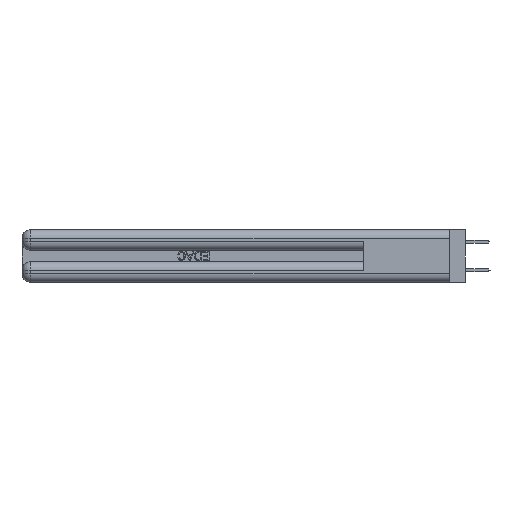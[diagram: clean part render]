
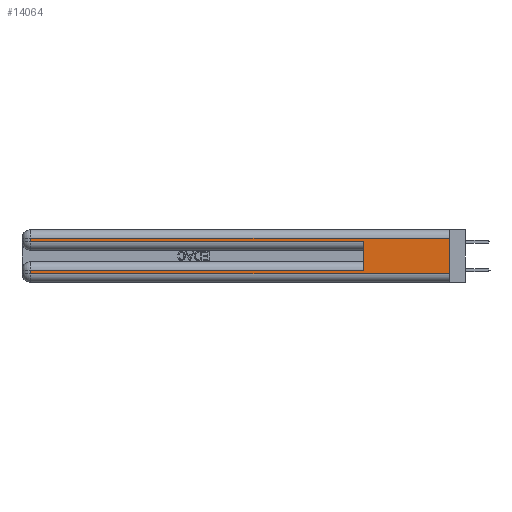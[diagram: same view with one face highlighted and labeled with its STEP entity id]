
A CAD part, left-side view. The second image highlights one B-rep face of the part: STEP entity #14064.
In plain terms, the highlighted planar face has unit normal (-1, 0, 0).
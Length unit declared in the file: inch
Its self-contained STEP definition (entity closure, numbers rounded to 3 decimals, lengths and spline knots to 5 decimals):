
#361 = DIRECTION ( 'NONE',  ( 0., 0., -1. ) ) ;
#1210 = LINE ( 'NONE', #43359, #11063 ) ;
#1530 = CARTESIAN_POINT ( 'NONE',  ( 0., 2.94, 0.31 ) ) ;
#2411 = VERTEX_POINT ( 'NONE', #1530 ) ;
#2597 = CARTESIAN_POINT ( 'NONE',  ( 0., 0., 0.085 ) ) ;
#3445 = FACE_OUTER_BOUND ( 'NONE', #27791, .T. ) ;
#3610 = VECTOR ( 'NONE', #22589, 39.37008 ) ;
#5219 = CARTESIAN_POINT ( 'NONE',  ( 0., 2.94, 0.06 ) ) ;
#5865 = VECTOR ( 'NONE', #21682, 39.37008 ) ;
#6076 = CARTESIAN_POINT ( 'NONE',  ( 0., 2.94, 0.37 ) ) ;
#6816 = CARTESIAN_POINT ( 'NONE',  ( 0., 2.94, 0.085 ) ) ;
#7654 = PLANE ( 'NONE',  #24106 ) ;
#7671 = EDGE_CURVE ( 'NONE', #40199, #2411, #27266, .T. ) ;
#10002 = DIRECTION ( 'NONE',  ( 0., 0., -1. ) ) ;
#10071 = EDGE_CURVE ( 'NONE', #16472, #32196, #44572, .T. ) ;
#11063 = VECTOR ( 'NONE', #21598, 39.37008 ) ;
#11305 = CARTESIAN_POINT ( 'NONE',  ( 0., 0., 0.06 ) ) ;
#11540 = VERTEX_POINT ( 'NONE', #37155 ) ;
#13101 = ORIENTED_EDGE ( 'NONE', *, *, #10071, .T. ) ;
#14064 = ADVANCED_FACE ( 'NONE', ( #3445 ), #7654, .F. ) ;
#14538 = VECTOR ( 'NONE', #24795, 39.37008 ) ;
#14700 = ORIENTED_EDGE ( 'NONE', *, *, #30115, .T. ) ;
#15029 = CARTESIAN_POINT ( 'NONE',  ( 0., 0., 0.06 ) ) ;
#15104 = CARTESIAN_POINT ( 'NONE',  ( 0., 0.6, 0.145 ) ) ;
#15451 = VECTOR ( 'NONE', #10002, 39.37008 ) ;
#15747 = LINE ( 'NONE', #6076, #5865 ) ;
#16456 = LINE ( 'NONE', #36750, #26255 ) ;
#16472 = VERTEX_POINT ( 'NONE', #6816 ) ;
#18635 = VECTOR ( 'NONE', #26447, 39.37008 ) ;
#18998 = EDGE_CURVE ( 'NONE', #2411, #11540, #15747, .T. ) ;
#21598 = DIRECTION ( 'NONE',  ( 0., 0., -1. ) ) ;
#21682 = DIRECTION ( 'NONE',  ( 0., 0., -1. ) ) ;
#22578 = DIRECTION ( 'NONE',  ( 1., 0., 0. ) ) ;
#22589 = DIRECTION ( 'NONE',  ( 0., 0., 1. ) ) ;
#23116 = VERTEX_POINT ( 'NONE', #46490 ) ;
#24106 = AXIS2_PLACEMENT_3D ( 'NONE', #44316, #22578, #361 ) ;
#24795 = DIRECTION ( 'NONE',  ( 0., 1., 0. ) ) ;
#26255 = VECTOR ( 'NONE', #33243, 39.37008 ) ;
#26256 = CARTESIAN_POINT ( 'NONE',  ( 0., 0.6, 0.085 ) ) ;
#26447 = DIRECTION ( 'NONE',  ( 0., 1., 0. ) ) ;
#27266 = LINE ( 'NONE', #33800, #18635 ) ;
#27475 = VERTEX_POINT ( 'NONE', #26256 ) ;
#27791 = EDGE_LOOP ( 'NONE', ( #36789, #45440, #37292, #37351, #36656, #14700, #13101, #35367 ) ) ;
#28135 = EDGE_CURVE ( 'NONE', #32196, #33155, #42498, .T. ) ;
#28442 = CARTESIAN_POINT ( 'NONE',  ( 0., 2.94, 0.37 ) ) ;
#30115 = EDGE_CURVE ( 'NONE', #27475, #16472, #42592, .T. ) ;
#30184 = EDGE_CURVE ( 'NONE', #40199, #33155, #1210, .T. ) ;
#32196 = VERTEX_POINT ( 'NONE', #5219 ) ;
#32887 = VECTOR ( 'NONE', #37051, 39.37008 ) ;
#33155 = VERTEX_POINT ( 'NONE', #11305 ) ;
#33243 = DIRECTION ( 'NONE',  ( 0., -1., 0. ) ) ;
#33800 = CARTESIAN_POINT ( 'NONE',  ( 0., 0., 0.31 ) ) ;
#34909 = CARTESIAN_POINT ( 'NONE',  ( 0., 0., 0.31 ) ) ;
#35367 = ORIENTED_EDGE ( 'NONE', *, *, #28135, .T. ) ;
#36656 = ORIENTED_EDGE ( 'NONE', *, *, #44208, .F. ) ;
#36750 = CARTESIAN_POINT ( 'NONE',  ( 0., 0., 0.285 ) ) ;
#36789 = ORIENTED_EDGE ( 'NONE', *, *, #30184, .F. ) ;
#37051 = DIRECTION ( 'NONE',  ( 0., -1., 0. ) ) ;
#37155 = CARTESIAN_POINT ( 'NONE',  ( 0., 2.94, 0.285 ) ) ;
#37292 = ORIENTED_EDGE ( 'NONE', *, *, #18998, .T. ) ;
#37351 = ORIENTED_EDGE ( 'NONE', *, *, #39297, .T. ) ;
#39297 = EDGE_CURVE ( 'NONE', #11540, #23116, #16456, .T. ) ;
#40199 = VERTEX_POINT ( 'NONE', #34909 ) ;
#42498 = LINE ( 'NONE', #15029, #32887 ) ;
#42592 = LINE ( 'NONE', #2597, #14538 ) ;
#42673 = LINE ( 'NONE', #15104, #3610 ) ;
#43359 = CARTESIAN_POINT ( 'NONE',  ( 0., 0., 0.37 ) ) ;
#44208 = EDGE_CURVE ( 'NONE', #27475, #23116, #42673, .T. ) ;
#44316 = CARTESIAN_POINT ( 'NONE',  ( 0., 0., 0.37 ) ) ;
#44572 = LINE ( 'NONE', #28442, #15451 ) ;
#45440 = ORIENTED_EDGE ( 'NONE', *, *, #7671, .T. ) ;
#46490 = CARTESIAN_POINT ( 'NONE',  ( 0., 0.6, 0.285 ) ) ;
